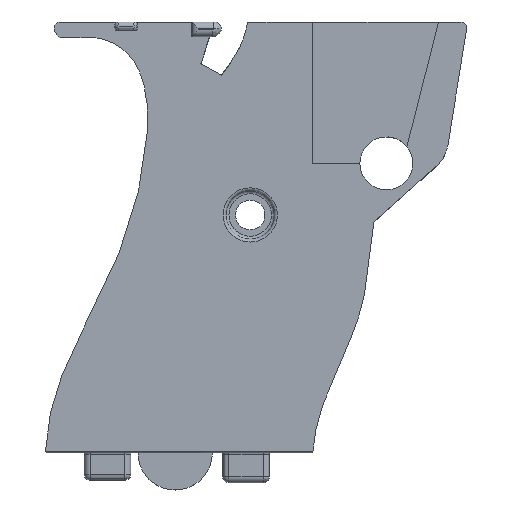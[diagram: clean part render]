
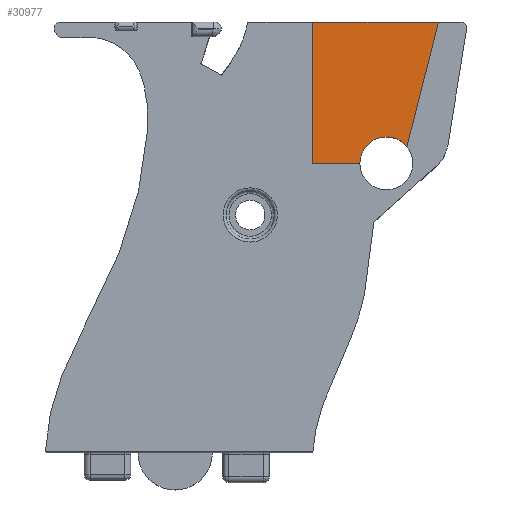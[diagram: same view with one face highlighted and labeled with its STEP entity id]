
A CAD part, top view. The second image highlights one B-rep face of the part: STEP entity #30977.
In plain terms, the highlighted planar face has unit normal (0, 0, 1).
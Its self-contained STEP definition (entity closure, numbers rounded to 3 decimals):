
#426=CIRCLE('',#31382,4.492);
#759=PLANE('',#31399);
#2430=FACE_OUTER_BOUND('',#4214,.T.);
#4214=EDGE_LOOP('',(#27793,#27794,#27795,#27796,#27797));
#5957=LINE('',#61368,#7774);
#6025=LINE('',#63244,#7842);
#6034=LINE('',#63532,#7851);
#6035=LINE('',#63534,#7852);
#7774=VECTOR('',#33714,10.);
#7842=VECTOR('',#33914,10.);
#7851=VECTOR('',#33959,10.);
#7852=VECTOR('',#33962,10.);
#13517=VERTEX_POINT('',#61365);
#13518=VERTEX_POINT('',#61367);
#13638=VERTEX_POINT('',#63241);
#13639=VERTEX_POINT('',#63243);
#13640=VERTEX_POINT('',#63247);
#18146=EDGE_CURVE('',#13517,#13518,#5957,.T.);
#18353=EDGE_CURVE('',#13638,#13639,#6025,.T.);
#18356=EDGE_CURVE('',#13640,#13638,#426,.T.);
#18379=EDGE_CURVE('',#13518,#13640,#6034,.T.);
#18380=EDGE_CURVE('',#13639,#13517,#6035,.T.);
#27793=ORIENTED_EDGE('',*,*,#18380,.F.);
#27794=ORIENTED_EDGE('',*,*,#18353,.F.);
#27795=ORIENTED_EDGE('',*,*,#18356,.F.);
#27796=ORIENTED_EDGE('',*,*,#18379,.F.);
#27797=ORIENTED_EDGE('',*,*,#18146,.F.);
#30977=ADVANCED_FACE('',(#2430),#759,.T.);
#31382=AXIS2_PLACEMENT_3D('',#63249,#33919,#33920);
#31399=AXIS2_PLACEMENT_3D('',#63533,#33960,#33961);
#33714=DIRECTION('',(1.,0.,0.));
#33914=DIRECTION('',(-1.,0.,0.));
#33919=DIRECTION('center_axis',(0.,0.,1.));
#33920=DIRECTION('ref_axis',(-1.,0.,0.));
#33959=DIRECTION('',(-0.245,-0.969,0.));
#33960=DIRECTION('center_axis',(0.,0.,1.));
#33961=DIRECTION('ref_axis',(-1.,0.,0.));
#33962=DIRECTION('',(0.,1.,0.));
#61365=CARTESIAN_POINT('',(-28.658,33.7,3.));
#61367=CARTESIAN_POINT('',(-7.335,33.7,3.));
#61368=CARTESIAN_POINT('',(-55.413,33.7,3.));
#63241=CARTESIAN_POINT('',(-20.656,9.741,3.));
#63243=CARTESIAN_POINT('',(-28.658,9.741,3.));
#63244=CARTESIAN_POINT('',(-20.656,9.741,3.));
#63247=CARTESIAN_POINT('',(-12.679,12.575,3.));
#63249=CARTESIAN_POINT('Origin',(-16.164,9.741,3.));
#63532=CARTESIAN_POINT('',(-7.335,33.7,3.));
#63533=CARTESIAN_POINT('Origin',(-38.264,-2.8,3.));
#63534=CARTESIAN_POINT('',(-28.658,33.7,3.));
